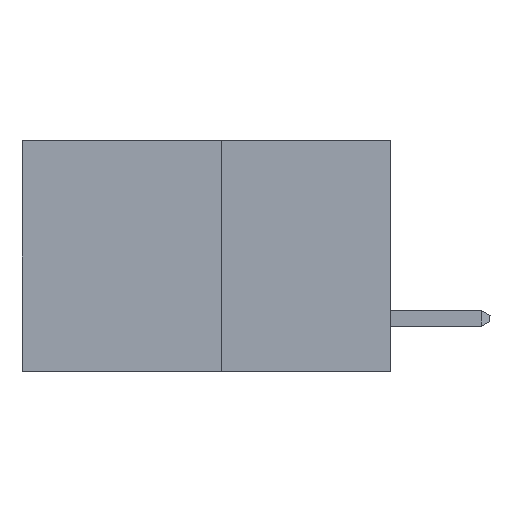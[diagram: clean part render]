
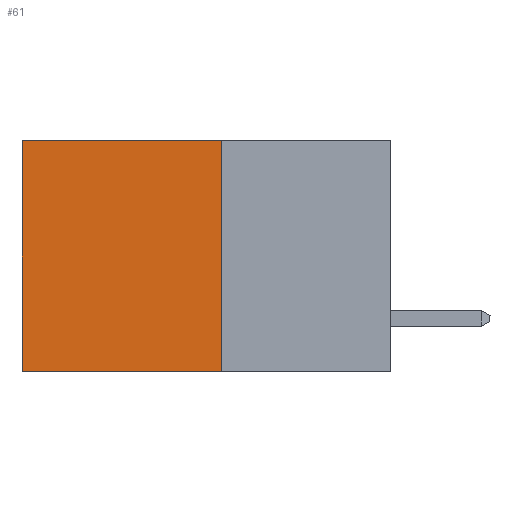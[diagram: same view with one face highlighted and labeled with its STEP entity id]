
A CAD part, left-side view. The second image highlights one B-rep face of the part: STEP entity #61.
In plain terms, the highlighted planar face has unit normal (-1, 0, 0).
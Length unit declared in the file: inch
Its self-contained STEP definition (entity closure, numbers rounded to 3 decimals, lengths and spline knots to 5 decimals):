
#61 = ADVANCED_FACE ( 'NONE', ( #23640 ), #23957, .F. ) ;
#983 = EDGE_CURVE ( 'NONE', #26014, #6827, #5884, .T. ) ;
#1918 = DIRECTION ( 'NONE',  ( 0., 0., -1. ) ) ;
#2890 = CARTESIAN_POINT ( 'NONE',  ( 0.277, 0.27, -0.37 ) ) ;
#3001 = CARTESIAN_POINT ( 'NONE',  ( 0.277, 0.27, -0.37 ) ) ;
#4555 = VECTOR ( 'NONE', #1918, 39.37008 ) ;
#5884 = LINE ( 'NONE', #3001, #4555 ) ;
#6827 = VERTEX_POINT ( 'NONE', #9760 ) ;
#7131 = DIRECTION ( 'NONE',  ( 0., 1., 0. ) ) ;
#7383 = EDGE_CURVE ( 'NONE', #6827, #12993, #10664, .T. ) ;
#8084 = EDGE_CURVE ( 'NONE', #26014, #26686, #15013, .T. ) ;
#8586 = LINE ( 'NONE', #24467, #19919 ) ;
#9760 = CARTESIAN_POINT ( 'NONE',  ( 0.277, 0.27, -0.37 ) ) ;
#10664 = LINE ( 'NONE', #2890, #22026 ) ;
#11470 = CARTESIAN_POINT ( 'NONE',  ( 0.277, 0.59, -0.37 ) ) ;
#12340 = EDGE_LOOP ( 'NONE', ( #26367, #18387, #24154, #25623 ) ) ;
#12993 = VERTEX_POINT ( 'NONE', #11470 ) ;
#15013 = LINE ( 'NONE', #15844, #25732 ) ;
#15071 = EDGE_CURVE ( 'NONE', #26686, #12993, #8586, .T. ) ;
#15844 = CARTESIAN_POINT ( 'NONE',  ( 0.277, 0.27, 0. ) ) ;
#16280 = AXIS2_PLACEMENT_3D ( 'NONE', #20792, #23921, #22465 ) ;
#18387 = ORIENTED_EDGE ( 'NONE', *, *, #7383, .F. ) ;
#18775 = CARTESIAN_POINT ( 'NONE',  ( 0.277, 0.59, 0. ) ) ;
#19919 = VECTOR ( 'NONE', #26601, 39.37008 ) ;
#20792 = CARTESIAN_POINT ( 'NONE',  ( 0.277, 0.27, -0.37 ) ) ;
#22026 = VECTOR ( 'NONE', #7131, 39.37008 ) ;
#22287 = DIRECTION ( 'NONE',  ( 0., 1., 0. ) ) ;
#22465 = DIRECTION ( 'NONE',  ( 0., 0., -1. ) ) ;
#23106 = CARTESIAN_POINT ( 'NONE',  ( 0.277, 0.27, 0. ) ) ;
#23640 = FACE_OUTER_BOUND ( 'NONE', #12340, .T. ) ;
#23921 = DIRECTION ( 'NONE',  ( 1., 0., 0. ) ) ;
#23957 = PLANE ( 'NONE',  #16280 ) ;
#24154 = ORIENTED_EDGE ( 'NONE', *, *, #983, .F. ) ;
#24467 = CARTESIAN_POINT ( 'NONE',  ( 0.277, 0.59, -0.37 ) ) ;
#25623 = ORIENTED_EDGE ( 'NONE', *, *, #8084, .T. ) ;
#25732 = VECTOR ( 'NONE', #22287, 39.37008 ) ;
#26014 = VERTEX_POINT ( 'NONE', #23106 ) ;
#26367 = ORIENTED_EDGE ( 'NONE', *, *, #15071, .T. ) ;
#26601 = DIRECTION ( 'NONE',  ( 0., 0., -1. ) ) ;
#26686 = VERTEX_POINT ( 'NONE', #18775 ) ;
